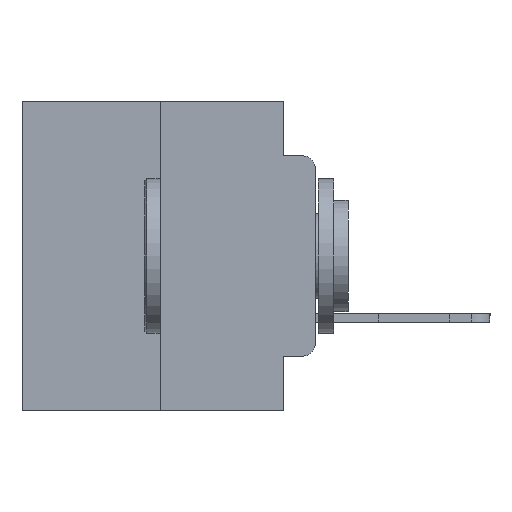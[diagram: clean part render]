
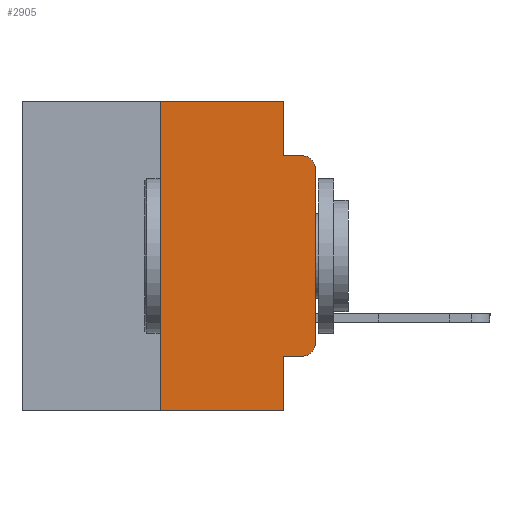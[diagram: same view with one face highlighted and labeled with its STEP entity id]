
A CAD part, left-side view. The second image highlights one B-rep face of the part: STEP entity #2905.
In plain terms, the highlighted planar face has unit normal (-1, 0, 0).
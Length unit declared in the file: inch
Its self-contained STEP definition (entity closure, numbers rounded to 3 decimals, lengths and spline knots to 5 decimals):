
#80 = ORIENTED_EDGE ( 'NONE', *, *, #443, .T. ) ;
#443 = EDGE_CURVE ( 'NONE', #24362, #20800, #22172, .T. ) ;
#802 = ORIENTED_EDGE ( 'NONE', *, *, #1416, .F. ) ;
#1029 = VERTEX_POINT ( 'NONE', #24621 ) ;
#1223 = EDGE_CURVE ( 'NONE', #8562, #18301, #15370, .T. ) ;
#1263 = EDGE_CURVE ( 'NONE', #18301, #1305, #20072, .T. ) ;
#1277 = EDGE_CURVE ( 'NONE', #22400, #1305, #18841, .T. ) ;
#1305 = VERTEX_POINT ( 'NONE', #5582 ) ;
#1328 = EDGE_CURVE ( 'NONE', #1029, #22400, #11569, .T. ) ;
#1366 = EDGE_CURVE ( 'NONE', #24362, #1633, #4638, .T. ) ;
#1416 = EDGE_CURVE ( 'NONE', #19257, #20800, #24131, .T. ) ;
#1463 = EDGE_CURVE ( 'NONE', #19257, #8058, #22399, .T. ) ;
#1561 = EDGE_CURVE ( 'NONE', #8058, #8562, #18153, .T. ) ;
#1633 = VERTEX_POINT ( 'NONE', #12228 ) ;
#2118 = VECTOR ( 'NONE', #8869, 39.37008 ) ;
#2770 = CARTESIAN_POINT ( 'NONE',  ( 0., 0.051, -0.0885 ) ) ;
#2905 = ADVANCED_FACE ( 'NONE', ( #14324 ), #9658, .F. ) ;
#3176 = LINE ( 'NONE', #4446, #18487 ) ;
#3273 = DIRECTION ( 'NONE',  ( 0., -1., 0. ) ) ;
#3600 = CARTESIAN_POINT ( 'NONE',  ( 0., 0.25, -0.5 ) ) ;
#3633 = DIRECTION ( 'NONE',  ( -1., 0., 0. ) ) ;
#3660 = CARTESIAN_POINT ( 'NONE',  ( 0., 0.02, -0.1085 ) ) ;
#3884 = DIRECTION ( 'NONE',  ( 0., 0., 1. ) ) ;
#4446 = CARTESIAN_POINT ( 'NONE',  ( 0., 0.473, 0. ) ) ;
#4638 = LINE ( 'NONE', #6317, #22096 ) ;
#5582 = CARTESIAN_POINT ( 'NONE',  ( 0., 0.02, -0.0885 ) ) ;
#6317 = CARTESIAN_POINT ( 'NONE',  ( 0., 0.25, 0. ) ) ;
#6670 = DIRECTION ( 'NONE',  ( 0., -1., 0. ) ) ;
#6878 = DIRECTION ( 'NONE',  ( 0., 0., 1. ) ) ;
#6883 = CARTESIAN_POINT ( 'NONE',  ( 0., 0.051, 0. ) ) ;
#6926 = ORIENTED_EDGE ( 'NONE', *, *, #1277, .F. ) ;
#7600 = AXIS2_PLACEMENT_3D ( 'NONE', #3660, #3633, #8641 ) ;
#7772 = EDGE_LOOP ( 'NONE', ( #18048, #21970, #6926, #19330, #12201, #15594, #80, #802, #12390, #13042 ) ) ;
#8058 = VERTEX_POINT ( 'NONE', #9023 ) ;
#8413 = VECTOR ( 'NONE', #26225, 39.37008 ) ;
#8562 = VERTEX_POINT ( 'NONE', #24318 ) ;
#8641 = DIRECTION ( 'NONE',  ( 0., 0., -1. ) ) ;
#8869 = DIRECTION ( 'NONE',  ( 0., -1., 0. ) ) ;
#9023 = CARTESIAN_POINT ( 'NONE',  ( 0., 0.02, -0.4115 ) ) ;
#9658 = PLANE ( 'NONE',  #20335 ) ;
#10751 = CARTESIAN_POINT ( 'NONE',  ( 0., 0.051, -0.5 ) ) ;
#10971 = CARTESIAN_POINT ( 'NONE',  ( 0., 0.473, -0.5 ) ) ;
#11569 = LINE ( 'NONE', #6883, #21520 ) ;
#12201 = ORIENTED_EDGE ( 'NONE', *, *, #21399, .F. ) ;
#12228 = CARTESIAN_POINT ( 'NONE',  ( 0., 0.25, 0. ) ) ;
#12377 = CARTESIAN_POINT ( 'NONE',  ( 0., 0., -0.1085 ) ) ;
#12390 = ORIENTED_EDGE ( 'NONE', *, *, #1463, .T. ) ;
#13042 = ORIENTED_EDGE ( 'NONE', *, *, #1561, .T. ) ;
#13279 = DIRECTION ( 'NONE',  ( 0., 0., -1. ) ) ;
#14013 = CARTESIAN_POINT ( 'NONE',  ( 0., 0.051, -0.4115 ) ) ;
#14324 = FACE_OUTER_BOUND ( 'NONE', #7772, .T. ) ;
#14768 = VECTOR ( 'NONE', #3884, 39.37008 ) ;
#15370 = LINE ( 'NONE', #24121, #14768 ) ;
#15594 = ORIENTED_EDGE ( 'NONE', *, *, #1366, .F. ) ;
#15722 = VECTOR ( 'NONE', #3273, 39.37008 ) ;
#17238 = DIRECTION ( 'NONE',  ( 0., 0., -1. ) ) ;
#17409 = DIRECTION ( 'NONE',  ( -1., 0., 0. ) ) ;
#17473 = CARTESIAN_POINT ( 'NONE',  ( 0., 0.02, -0.3915 ) ) ;
#17794 = DIRECTION ( 'NONE',  ( 0., 0., -1. ) ) ;
#18048 = ORIENTED_EDGE ( 'NONE', *, *, #1223, .T. ) ;
#18153 = CIRCLE ( 'NONE', #21858, 0.02 ) ;
#18301 = VERTEX_POINT ( 'NONE', #12377 ) ;
#18487 = VECTOR ( 'NONE', #6670, 39.37008 ) ;
#18509 = VECTOR ( 'NONE', #17794, 39.37008 ) ;
#18841 = LINE ( 'NONE', #2770, #2118 ) ;
#19257 = VERTEX_POINT ( 'NONE', #21264 ) ;
#19330 = ORIENTED_EDGE ( 'NONE', *, *, #1328, .F. ) ;
#19675 = CARTESIAN_POINT ( 'NONE',  ( 0., 0.051, 0. ) ) ;
#20072 = CIRCLE ( 'NONE', #7600, 0.02 ) ;
#20335 = AXIS2_PLACEMENT_3D ( 'NONE', #20912, #21333, #20753 ) ;
#20753 = DIRECTION ( 'NONE',  ( 0., 0., -1. ) ) ;
#20800 = VERTEX_POINT ( 'NONE', #10751 ) ;
#20912 = CARTESIAN_POINT ( 'NONE',  ( 0., 0.473, 0. ) ) ;
#21264 = CARTESIAN_POINT ( 'NONE',  ( 0., 0.051, -0.4115 ) ) ;
#21333 = DIRECTION ( 'NONE',  ( 1., 0., 0. ) ) ;
#21399 = EDGE_CURVE ( 'NONE', #1633, #1029, #3176, .T. ) ;
#21520 = VECTOR ( 'NONE', #13279, 39.37008 ) ;
#21858 = AXIS2_PLACEMENT_3D ( 'NONE', #17473, #17409, #17238 ) ;
#21970 = ORIENTED_EDGE ( 'NONE', *, *, #1263, .T. ) ;
#22096 = VECTOR ( 'NONE', #6878, 39.37008 ) ;
#22172 = LINE ( 'NONE', #10971, #15722 ) ;
#22399 = LINE ( 'NONE', #14013, #8413 ) ;
#22400 = VERTEX_POINT ( 'NONE', #25097 ) ;
#24121 = CARTESIAN_POINT ( 'NONE',  ( 0., 0., 0. ) ) ;
#24131 = LINE ( 'NONE', #19675, #18509 ) ;
#24318 = CARTESIAN_POINT ( 'NONE',  ( 0., 0., -0.3915 ) ) ;
#24362 = VERTEX_POINT ( 'NONE', #3600 ) ;
#24621 = CARTESIAN_POINT ( 'NONE',  ( 0., 0.051, 0. ) ) ;
#25097 = CARTESIAN_POINT ( 'NONE',  ( 0., 0.051, -0.0885 ) ) ;
#26225 = DIRECTION ( 'NONE',  ( 0., -1., 0. ) ) ;
